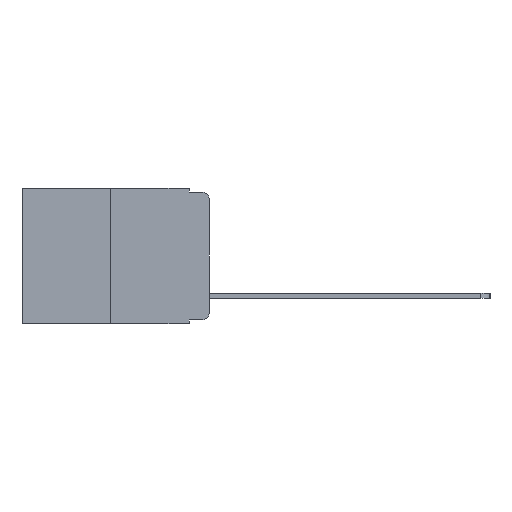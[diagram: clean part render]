
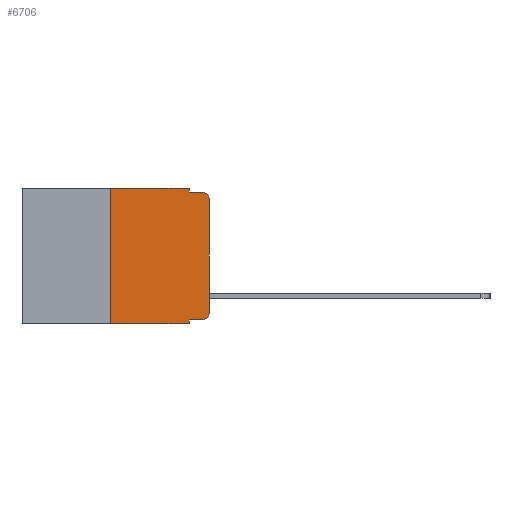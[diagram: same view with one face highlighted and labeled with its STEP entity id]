
A CAD part, left-side view. The second image highlights one B-rep face of the part: STEP entity #6706.
In plain terms, the highlighted planar face has unit normal (-1, 0, 0).
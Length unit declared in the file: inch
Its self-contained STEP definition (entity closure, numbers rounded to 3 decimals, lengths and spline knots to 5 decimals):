
#636 = EDGE_CURVE ( 'NONE', #10995, #11628, #18664, .T. ) ;
#995 = VERTEX_POINT ( 'NONE', #15595 ) ;
#1433 = VECTOR ( 'NONE', #19743, 39.37008 ) ;
#1500 = VECTOR ( 'NONE', #2822, 39.37008 ) ;
#2076 = LINE ( 'NONE', #10145, #1500 ) ;
#2092 = CARTESIAN_POINT ( 'NONE',  ( 0., 0., 0. ) ) ;
#2609 = DIRECTION ( 'NONE',  ( 0., -1., 0. ) ) ;
#2639 = DIRECTION ( 'NONE',  ( -1., 0., 0. ) ) ;
#2822 = DIRECTION ( 'NONE',  ( 0., 0., -1. ) ) ;
#3017 = VERTEX_POINT ( 'NONE', #18914 ) ;
#3300 = VERTEX_POINT ( 'NONE', #7267 ) ;
#3499 = ORIENTED_EDGE ( 'NONE', *, *, #15738, .T. ) ;
#3564 = EDGE_CURVE ( 'NONE', #995, #10483, #20636, .T. ) ;
#3748 = CARTESIAN_POINT ( 'NONE',  ( 0., 0.051, 0. ) ) ;
#4208 = VECTOR ( 'NONE', #9486, 39.37008 ) ;
#4302 = ORIENTED_EDGE ( 'NONE', *, *, #12118, .F. ) ;
#5127 = LINE ( 'NONE', #7666, #20061 ) ;
#5163 = VERTEX_POINT ( 'NONE', #3748 ) ;
#5417 = CARTESIAN_POINT ( 'NONE',  ( 0., 0.051, -0.333 ) ) ;
#5496 = CARTESIAN_POINT ( 'NONE',  ( 0., 0.02, -0.03 ) ) ;
#6277 = VECTOR ( 'NONE', #15829, 39.37008 ) ;
#6280 = VERTEX_POINT ( 'NONE', #7304 ) ;
#6706 = ADVANCED_FACE ( 'NONE', ( #14075 ), #22438, .F. ) ;
#7135 = EDGE_LOOP ( 'NONE', ( #21123, #15229, #10391, #21743, #4302, #12242, #15233, #9144, #3499, #19783 ) ) ;
#7267 = CARTESIAN_POINT ( 'NONE',  ( 0., 0.02, -0.01 ) ) ;
#7303 = DIRECTION ( 'NONE',  ( 0., 0., -1. ) ) ;
#7304 = CARTESIAN_POINT ( 'NONE',  ( 0., 0.051, -0.01 ) ) ;
#7666 = CARTESIAN_POINT ( 'NONE',  ( 0., 0.473, -0.343 ) ) ;
#8334 = CARTESIAN_POINT ( 'NONE',  ( 0., 0., -0.313 ) ) ;
#9097 = LINE ( 'NONE', #22331, #22223 ) ;
#9103 = VECTOR ( 'NONE', #22107, 39.37008 ) ;
#9108 = CARTESIAN_POINT ( 'NONE',  ( 0., 0.25, -0.343 ) ) ;
#9144 = ORIENTED_EDGE ( 'NONE', *, *, #3564, .F. ) ;
#9486 = DIRECTION ( 'NONE',  ( 0., -1., 0. ) ) ;
#9968 = CIRCLE ( 'NONE', #21552, 0.02 ) ;
#10045 = CARTESIAN_POINT ( 'NONE',  ( 0., 0.25, 0. ) ) ;
#10145 = CARTESIAN_POINT ( 'NONE',  ( 0., 0.051, 0. ) ) ;
#10176 = LINE ( 'NONE', #11294, #4208 ) ;
#10391 = ORIENTED_EDGE ( 'NONE', *, *, #17951, .F. ) ;
#10483 = VERTEX_POINT ( 'NONE', #15960 ) ;
#10995 = VERTEX_POINT ( 'NONE', #8334 ) ;
#11294 = CARTESIAN_POINT ( 'NONE',  ( 0., 0.051, -0.01 ) ) ;
#11628 = VERTEX_POINT ( 'NONE', #13847 ) ;
#12118 = EDGE_CURVE ( 'NONE', #21787, #5163, #9097, .T. ) ;
#12160 = CIRCLE ( 'NONE', #20430, 0.02 ) ;
#12242 = ORIENTED_EDGE ( 'NONE', *, *, #14827, .F. ) ;
#13090 = AXIS2_PLACEMENT_3D ( 'NONE', #17216, #17012, #16680 ) ;
#13535 = CARTESIAN_POINT ( 'NONE',  ( 0., 0.02, -0.313 ) ) ;
#13847 = CARTESIAN_POINT ( 'NONE',  ( 0., 0., -0.03 ) ) ;
#14075 = FACE_OUTER_BOUND ( 'NONE', #7135, .T. ) ;
#14387 = EDGE_CURVE ( 'NONE', #5163, #6280, #2076, .T. ) ;
#14827 = EDGE_CURVE ( 'NONE', #23025, #21787, #20134, .T. ) ;
#15229 = ORIENTED_EDGE ( 'NONE', *, *, #15756, .T. ) ;
#15233 = ORIENTED_EDGE ( 'NONE', *, *, #16215, .T. ) ;
#15355 = DIRECTION ( 'NONE',  ( 0., 0., -1. ) ) ;
#15416 = VECTOR ( 'NONE', #16911, 39.37008 ) ;
#15595 = CARTESIAN_POINT ( 'NONE',  ( 0., 0.051, -0.333 ) ) ;
#15738 = EDGE_CURVE ( 'NONE', #995, #3017, #20643, .T. ) ;
#15756 = EDGE_CURVE ( 'NONE', #11628, #3300, #9968, .T. ) ;
#15829 = DIRECTION ( 'NONE',  ( 0., 0., -1. ) ) ;
#15879 = CARTESIAN_POINT ( 'NONE',  ( 0., 0.051, 0. ) ) ;
#15960 = CARTESIAN_POINT ( 'NONE',  ( 0., 0.051, -0.343 ) ) ;
#16215 = EDGE_CURVE ( 'NONE', #23025, #10483, #5127, .T. ) ;
#16680 = DIRECTION ( 'NONE',  ( 0., 0., -1. ) ) ;
#16911 = DIRECTION ( 'NONE',  ( 0., 0., 1. ) ) ;
#17012 = DIRECTION ( 'NONE',  ( 1., 0., 0. ) ) ;
#17216 = CARTESIAN_POINT ( 'NONE',  ( 0., 0.473, 0. ) ) ;
#17951 = EDGE_CURVE ( 'NONE', #6280, #3300, #10176, .T. ) ;
#18096 = DIRECTION ( 'NONE',  ( -1., 0., 0. ) ) ;
#18107 = EDGE_CURVE ( 'NONE', #3017, #10995, #12160, .T. ) ;
#18664 = LINE ( 'NONE', #2092, #9103 ) ;
#18914 = CARTESIAN_POINT ( 'NONE',  ( 0., 0.02, -0.333 ) ) ;
#19743 = DIRECTION ( 'NONE',  ( 0., -1., 0. ) ) ;
#19783 = ORIENTED_EDGE ( 'NONE', *, *, #18107, .T. ) ;
#20061 = VECTOR ( 'NONE', #20247, 39.37008 ) ;
#20134 = LINE ( 'NONE', #22135, #15416 ) ;
#20247 = DIRECTION ( 'NONE',  ( 0., -1., 0. ) ) ;
#20430 = AXIS2_PLACEMENT_3D ( 'NONE', #13535, #2639, #15355 ) ;
#20636 = LINE ( 'NONE', #15879, #6277 ) ;
#20643 = LINE ( 'NONE', #5417, #1433 ) ;
#21123 = ORIENTED_EDGE ( 'NONE', *, *, #636, .T. ) ;
#21552 = AXIS2_PLACEMENT_3D ( 'NONE', #5496, #18096, #7303 ) ;
#21743 = ORIENTED_EDGE ( 'NONE', *, *, #14387, .F. ) ;
#21787 = VERTEX_POINT ( 'NONE', #10045 ) ;
#22107 = DIRECTION ( 'NONE',  ( 0., 0., 1. ) ) ;
#22135 = CARTESIAN_POINT ( 'NONE',  ( 0., 0.25, 0. ) ) ;
#22223 = VECTOR ( 'NONE', #2609, 39.37008 ) ;
#22331 = CARTESIAN_POINT ( 'NONE',  ( 0., 0.473, 0. ) ) ;
#22438 = PLANE ( 'NONE',  #13090 ) ;
#23025 = VERTEX_POINT ( 'NONE', #9108 ) ;
